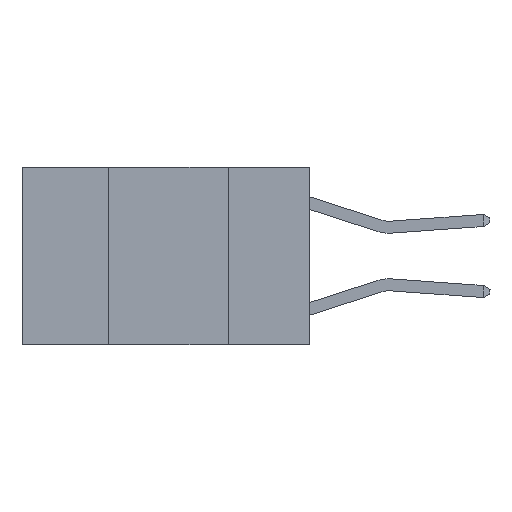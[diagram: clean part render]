
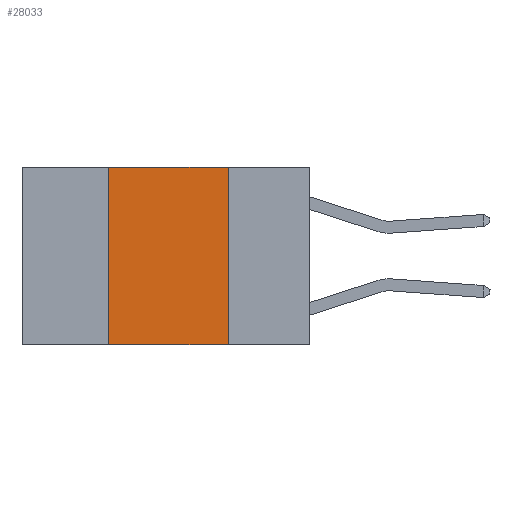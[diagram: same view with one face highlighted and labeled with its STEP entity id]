
A CAD part, left-side view. The second image highlights one B-rep face of the part: STEP entity #28033.
In plain terms, the highlighted planar face has unit normal (-1, 0, 0).
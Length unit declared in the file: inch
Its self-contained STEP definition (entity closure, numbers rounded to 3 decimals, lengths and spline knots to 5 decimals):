
#424 = EDGE_CURVE ( 'NONE', #20675, #4379, #31087, .T. ) ;
#1012 = VECTOR ( 'NONE', #32349, 39.37008 ) ;
#2886 = ORIENTED_EDGE ( 'NONE', *, *, #19527, .F. ) ;
#4379 = VERTEX_POINT ( 'NONE', #16238 ) ;
#4735 = CARTESIAN_POINT ( 'NONE',  ( 0., 0.17, 0. ) ) ;
#6911 = VECTOR ( 'NONE', #27725, 39.37008 ) ;
#7508 = DIRECTION ( 'NONE',  ( 0., 0., 1. ) ) ;
#9588 = FACE_OUTER_BOUND ( 'NONE', #22683, .T. ) ;
#11091 = EDGE_CURVE ( 'NONE', #20675, #20679, #24485, .T. ) ;
#12243 = AXIS2_PLACEMENT_3D ( 'NONE', #14109, #32522, #22168 ) ;
#13365 = VECTOR ( 'NONE', #16957, 39.37008 ) ;
#14109 = CARTESIAN_POINT ( 'NONE',  ( 0., 0.6, 0. ) ) ;
#15726 = ORIENTED_EDGE ( 'NONE', *, *, #25920, .F. ) ;
#16238 = CARTESIAN_POINT ( 'NONE',  ( 0., 0.42, 0. ) ) ;
#16953 = CARTESIAN_POINT ( 'NONE',  ( 0., 0.6, 0. ) ) ;
#16957 = DIRECTION ( 'NONE',  ( 0., -1., 0. ) ) ;
#19527 = EDGE_CURVE ( 'NONE', #4379, #26808, #19805, .T. ) ;
#19805 = LINE ( 'NONE', #16953, #1012 ) ;
#20061 = ORIENTED_EDGE ( 'NONE', *, *, #424, .F. ) ;
#20675 = VERTEX_POINT ( 'NONE', #23989 ) ;
#20679 = VERTEX_POINT ( 'NONE', #29346 ) ;
#22003 = PLANE ( 'NONE',  #12243 ) ;
#22168 = DIRECTION ( 'NONE',  ( 0., 0., -1. ) ) ;
#22683 = EDGE_LOOP ( 'NONE', ( #15726, #2886, #20061, #24832 ) ) ;
#23989 = CARTESIAN_POINT ( 'NONE',  ( 0., 0.42, -0.37 ) ) ;
#24485 = LINE ( 'NONE', #29685, #13365 ) ;
#24832 = ORIENTED_EDGE ( 'NONE', *, *, #11091, .T. ) ;
#25920 = EDGE_CURVE ( 'NONE', #26808, #20679, #32760, .T. ) ;
#26808 = VERTEX_POINT ( 'NONE', #4735 ) ;
#27725 = DIRECTION ( 'NONE',  ( 0., 0., -1. ) ) ;
#28033 = ADVANCED_FACE ( 'NONE', ( #9588 ), #22003, .F. ) ;
#28586 = CARTESIAN_POINT ( 'NONE',  ( 0., 0.42, 0. ) ) ;
#28733 = VECTOR ( 'NONE', #7508, 39.37008 ) ;
#29346 = CARTESIAN_POINT ( 'NONE',  ( 0., 0.17, -0.37 ) ) ;
#29685 = CARTESIAN_POINT ( 'NONE',  ( 0., 0.6, -0.37 ) ) ;
#30908 = CARTESIAN_POINT ( 'NONE',  ( 0., 0.17, 0. ) ) ;
#31087 = LINE ( 'NONE', #28586, #28733 ) ;
#32349 = DIRECTION ( 'NONE',  ( 0., -1., 0. ) ) ;
#32522 = DIRECTION ( 'NONE',  ( 1., 0., 0. ) ) ;
#32760 = LINE ( 'NONE', #30908, #6911 ) ;
